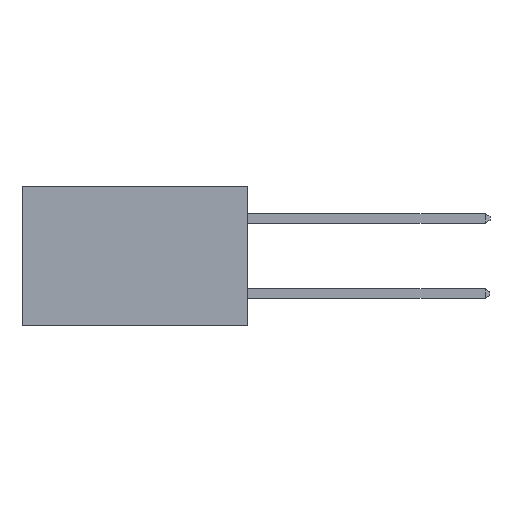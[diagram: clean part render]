
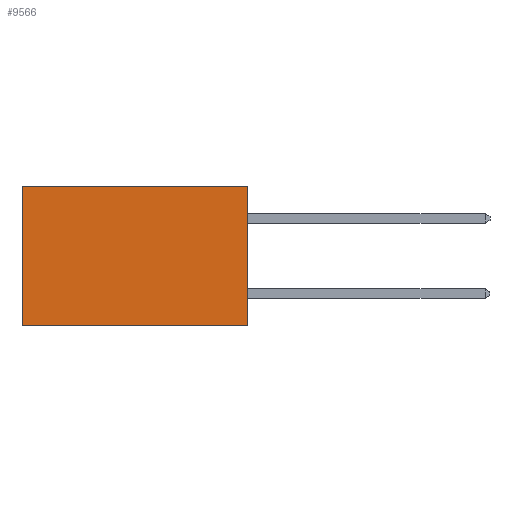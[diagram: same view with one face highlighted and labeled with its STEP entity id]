
A CAD part, left-side view. The second image highlights one B-rep face of the part: STEP entity #9566.
In plain terms, the highlighted planar face has unit normal (-1, 0, 0).
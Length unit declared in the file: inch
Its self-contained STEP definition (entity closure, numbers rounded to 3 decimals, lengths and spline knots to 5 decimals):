
#126 = DIRECTION ( 'NONE',  ( 0., 0., -1. ) ) ;
#226 = VECTOR ( 'NONE', #15723, 39.37008 ) ;
#704 = LINE ( 'NONE', #10693, #13193 ) ;
#1183 = CARTESIAN_POINT ( 'NONE',  ( 0.298, 0., 0. ) ) ;
#1704 = CARTESIAN_POINT ( 'NONE',  ( 0.298, 0.6, 0. ) ) ;
#2469 = VERTEX_POINT ( 'NONE', #7472 ) ;
#2721 = ORIENTED_EDGE ( 'NONE', *, *, #10778, .T. ) ;
#2909 = DIRECTION ( 'NONE',  ( 0., 1., 0. ) ) ;
#3667 = ORIENTED_EDGE ( 'NONE', *, *, #11192, .F. ) ;
#3802 = DIRECTION ( 'NONE',  ( 1., 0., 0. ) ) ;
#4492 = ORIENTED_EDGE ( 'NONE', *, *, #19552, .T. ) ;
#4955 = VERTEX_POINT ( 'NONE', #1704 ) ;
#4979 = VERTEX_POINT ( 'NONE', #14062 ) ;
#5292 = PLANE ( 'NONE',  #13285 ) ;
#5675 = CARTESIAN_POINT ( 'NONE',  ( 0.298, 0., -0.37 ) ) ;
#7472 = CARTESIAN_POINT ( 'NONE',  ( 0.298, 0.6, -0.37 ) ) ;
#8637 = LINE ( 'NONE', #9654, #226 ) ;
#9566 = ADVANCED_FACE ( 'NONE', ( #10373 ), #5292, .F. ) ;
#9585 = CARTESIAN_POINT ( 'NONE',  ( 0.298, 0., 0. ) ) ;
#9621 = VECTOR ( 'NONE', #126, 39.37008 ) ;
#9654 = CARTESIAN_POINT ( 'NONE',  ( 0.298, 0.6, 0. ) ) ;
#10373 = FACE_OUTER_BOUND ( 'NONE', #17427, .T. ) ;
#10685 = ORIENTED_EDGE ( 'NONE', *, *, #10743, .F. ) ;
#10693 = CARTESIAN_POINT ( 'NONE',  ( 0.298, 0., -0.37 ) ) ;
#10743 = EDGE_CURVE ( 'NONE', #4979, #12762, #17278, .T. ) ;
#10778 = EDGE_CURVE ( 'NONE', #4955, #2469, #8637, .T. ) ;
#11192 = EDGE_CURVE ( 'NONE', #12762, #2469, #704, .T. ) ;
#11817 = VECTOR ( 'NONE', #16759, 39.37008 ) ;
#12762 = VERTEX_POINT ( 'NONE', #5675 ) ;
#13193 = VECTOR ( 'NONE', #2909, 39.37008 ) ;
#13285 = AXIS2_PLACEMENT_3D ( 'NONE', #19163, #3802, #14646 ) ;
#14062 = CARTESIAN_POINT ( 'NONE',  ( 0.298, 0., 0. ) ) ;
#14646 = DIRECTION ( 'NONE',  ( 0., 0., -1. ) ) ;
#15723 = DIRECTION ( 'NONE',  ( 0., 0., -1. ) ) ;
#15866 = LINE ( 'NONE', #1183, #11817 ) ;
#16759 = DIRECTION ( 'NONE',  ( 0., 1., 0. ) ) ;
#17278 = LINE ( 'NONE', #9585, #9621 ) ;
#17427 = EDGE_LOOP ( 'NONE', ( #2721, #3667, #10685, #4492 ) ) ;
#19163 = CARTESIAN_POINT ( 'NONE',  ( 0.298, 0., 0. ) ) ;
#19552 = EDGE_CURVE ( 'NONE', #4979, #4955, #15866, .T. ) ;
